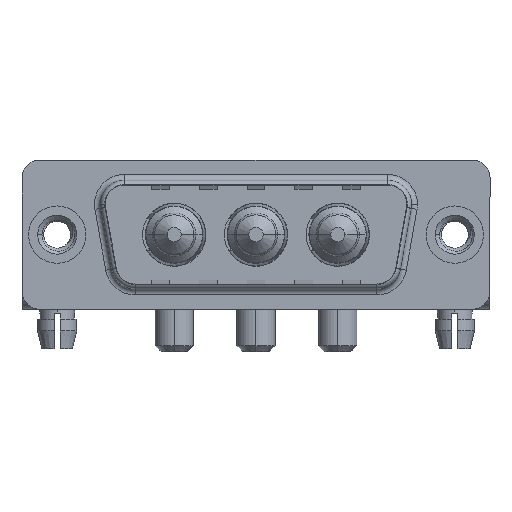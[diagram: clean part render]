
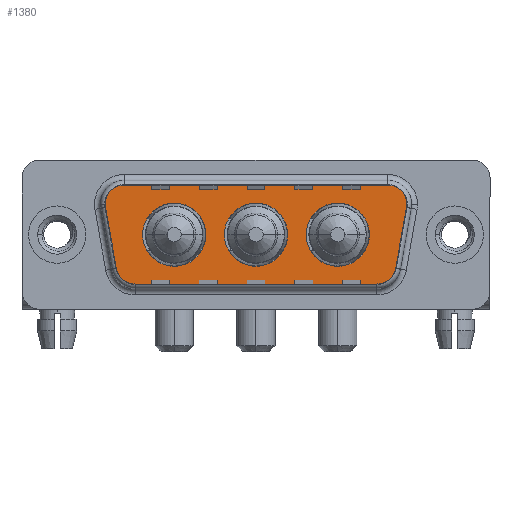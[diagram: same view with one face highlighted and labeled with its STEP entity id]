
A CAD part, top view. The second image highlights one B-rep face of the part: STEP entity #1380.
In plain terms, the highlighted planar face has unit normal (0, 0, 1).
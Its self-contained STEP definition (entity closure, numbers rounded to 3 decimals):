
#302 = DIRECTION ( 'NONE',  ( 0., 0., 1. ) ) ;
#380 = CARTESIAN_POINT ( 'NONE',  ( 26.866, -2.9, 0. ) ) ;
#477 = VECTOR ( 'NONE', #15163, 1000. ) ;
#493 = AXIS2_PLACEMENT_3D ( 'NONE', #7158, #10575, #11893 ) ;
#633 = VERTEX_POINT ( 'NONE', #14245 ) ;
#839 = EDGE_CURVE ( 'NONE', #13134, #1297, #13223, .T. ) ;
#893 = DIRECTION ( 'NONE',  ( -1., 0., 0. ) ) ;
#986 = DIRECTION ( 'NONE',  ( 1., 0., 0. ) ) ;
#1160 = VERTEX_POINT ( 'NONE', #13136 ) ;
#1214 = ORIENTED_EDGE ( 'NONE', *, *, #11689, .T. ) ;
#1252 = CIRCLE ( 'NONE', #4707, 2.65 ) ;
#1283 = DIRECTION ( 'NONE',  ( 0., 0., 1. ) ) ;
#1297 = VERTEX_POINT ( 'NONE', #1466 ) ;
#1345 = DIRECTION ( 'NONE',  ( 0., 0., 1. ) ) ;
#1366 = DIRECTION ( 'NONE',  ( 0., 0., 1. ) ) ;
#1380 = ADVANCED_FACE ( 'NONE', ( #2771, #7483, #3782, #6254 ), #10968, .T. ) ;
#1466 = CARTESIAN_POINT ( 'NONE',  ( 4.464, -3.247, 0. ) ) ;
#1900 = AXIS2_PLACEMENT_3D ( 'NONE', #6767, #10247, #986 ) ;
#2054 = ORIENTED_EDGE ( 'NONE', *, *, #5773, .F. ) ;
#2319 = VERTEX_POINT ( 'NONE', #10124 ) ;
#2365 = DIRECTION ( 'NONE',  ( 1., 0., 0. ) ) ;
#2606 = DIRECTION ( 'NONE',  ( 1., 0., 0. ) ) ;
#2658 = VECTOR ( 'NONE', #12943, 1000. ) ;
#2663 = DIRECTION ( 'NONE',  ( 0., 0., 1. ) ) ;
#2695 = ORIENTED_EDGE ( 'NONE', *, *, #8251, .F. ) ;
#2771 = FACE_BOUND ( 'NONE', #2846, .T. ) ;
#2846 = EDGE_LOOP ( 'NONE', ( #8643, #2695 ) ) ;
#3133 = CARTESIAN_POINT ( 'NONE',  ( 26.15, 0., 0. ) ) ;
#3180 = LINE ( 'NONE', #15089, #477 ) ;
#3241 = CARTESIAN_POINT ( 'NONE',  ( 14., 0., 0. ) ) ;
#3299 = EDGE_LOOP ( 'NONE', ( #7519, #13326, #3746, #1214, #10969, #6042, #6668, #4087, #4563 ) ) ;
#3429 = VERTEX_POINT ( 'NONE', #3133 ) ;
#3434 = VERTEX_POINT ( 'NONE', #14890 ) ;
#3510 = CARTESIAN_POINT ( 'NONE',  ( 9.8, 0., 0. ) ) ;
#3746 = ORIENTED_EDGE ( 'NONE', *, *, #10269, .T. ) ;
#3782 = FACE_BOUND ( 'NONE', #5805, .T. ) ;
#3991 = VECTOR ( 'NONE', #12380, 1000. ) ;
#4087 = ORIENTED_EDGE ( 'NONE', *, *, #6778, .T. ) ;
#4117 = AXIS2_PLACEMENT_3D ( 'NONE', #10049, #4189, #8894 ) ;
#4134 = CIRCLE ( 'NONE', #4387, 2.65 ) ;
#4189 = DIRECTION ( 'NONE',  ( 0., 0., 1. ) ) ;
#4387 = AXIS2_PLACEMENT_3D ( 'NONE', #14500, #2663, #6298 ) ;
#4513 = CIRCLE ( 'NONE', #9452, 2.65 ) ;
#4563 = ORIENTED_EDGE ( 'NONE', *, *, #6713, .T. ) ;
#4707 = AXIS2_PLACEMENT_3D ( 'NONE', #11364, #11443, #15074 ) ;
#5083 = AXIS2_PLACEMENT_3D ( 'NONE', #7715, #8865, #9946 ) ;
#5104 = CIRCLE ( 'NONE', #10549, 2.65 ) ;
#5110 = EDGE_CURVE ( 'NONE', #11005, #15207, #3180, .T. ) ;
#5317 = CARTESIAN_POINT ( 'NONE',  ( 29.859, 2.553, 0. ) ) ;
#5606 = CIRCLE ( 'NONE', #12028, 2. ) ;
#5612 = ORIENTED_EDGE ( 'NONE', *, *, #12303, .F. ) ;
#5619 = AXIS2_PLACEMENT_3D ( 'NONE', #10804, #302, #10657 ) ;
#5686 = DIRECTION ( 'NONE',  ( 0., 0., 1. ) ) ;
#5773 = EDGE_CURVE ( 'NONE', #3429, #2319, #13820, .T. ) ;
#5805 = EDGE_LOOP ( 'NONE', ( #7192, #5612 ) ) ;
#6042 = ORIENTED_EDGE ( 'NONE', *, *, #7007, .T. ) ;
#6254 = FACE_OUTER_BOUND ( 'NONE', #3299, .T. ) ;
#6298 = DIRECTION ( 'NONE',  ( 1., 0., 0. ) ) ;
#6511 = EDGE_CURVE ( 'NONE', #14499, #7944, #1252, .T. ) ;
#6583 = CIRCLE ( 'NONE', #4117, 2. ) ;
#6668 = ORIENTED_EDGE ( 'NONE', *, *, #839, .T. ) ;
#6713 = EDGE_CURVE ( 'NONE', #1160, #13533, #13273, .T. ) ;
#6767 = CARTESIAN_POINT ( 'NONE',  ( 5.411, 2.9, 0. ) ) ;
#6778 = EDGE_CURVE ( 'NONE', #1297, #1160, #10783, .T. ) ;
#6898 = LINE ( 'NONE', #14104, #2658 ) ;
#7007 = EDGE_CURVE ( 'NONE', #12529, #13134, #15237, .T. ) ;
#7013 = CARTESIAN_POINT ( 'NONE',  ( 6.434, -4.9, 0. ) ) ;
#7117 = EDGE_LOOP ( 'NONE', ( #2054, #9067 ) ) ;
#7158 = CARTESIAN_POINT ( 'NONE',  ( 23.5, 0., 0. ) ) ;
#7192 = ORIENTED_EDGE ( 'NONE', *, *, #7694, .F. ) ;
#7483 = FACE_BOUND ( 'NONE', #7117, .T. ) ;
#7519 = ORIENTED_EDGE ( 'NONE', *, *, #8624, .T. ) ;
#7694 = EDGE_CURVE ( 'NONE', #633, #3434, #4513, .T. ) ;
#7715 = CARTESIAN_POINT ( 'NONE',  ( 16.65, 0., 0. ) ) ;
#7944 = VERTEX_POINT ( 'NONE', #3241 ) ;
#8218 = DIRECTION ( 'NONE',  ( 1., 0., 0. ) ) ;
#8251 = EDGE_CURVE ( 'NONE', #7944, #14499, #11761, .T. ) ;
#8624 = EDGE_CURVE ( 'NONE', #13533, #11005, #11993, .T. ) ;
#8643 = ORIENTED_EDGE ( 'NONE', *, *, #6511, .F. ) ;
#8735 = CARTESIAN_POINT ( 'NONE',  ( 3.441, 2.553, 0. ) ) ;
#8807 = VECTOR ( 'NONE', #2606, 1000. ) ;
#8865 = DIRECTION ( 'NONE',  ( 0., 0., 1. ) ) ;
#8894 = DIRECTION ( 'NONE',  ( -1., 0., 0. ) ) ;
#9067 = ORIENTED_EDGE ( 'NONE', *, *, #12473, .F. ) ;
#9387 = DIRECTION ( 'NONE',  ( 1., 0., 0. ) ) ;
#9392 = VERTEX_POINT ( 'NONE', #14866 ) ;
#9397 = CARTESIAN_POINT ( 'NONE',  ( 9.8, 0., 0. ) ) ;
#9452 = AXIS2_PLACEMENT_3D ( 'NONE', #3510, #1345, #8218 ) ;
#9549 = CARTESIAN_POINT ( 'NONE',  ( 26.866, -2.9, 0. ) ) ;
#9691 = CARTESIAN_POINT ( 'NONE',  ( 3.441, 2.553, 0. ) ) ;
#9946 = DIRECTION ( 'NONE',  ( 1., 0., 0. ) ) ;
#9989 = CARTESIAN_POINT ( 'NONE',  ( 28.836, -3.247, 0. ) ) ;
#10049 = CARTESIAN_POINT ( 'NONE',  ( 27.889, 2.9, 0. ) ) ;
#10124 = CARTESIAN_POINT ( 'NONE',  ( 20.85, 0., 0. ) ) ;
#10152 = CARTESIAN_POINT ( 'NONE',  ( 5.411, 4.9, 0. ) ) ;
#10247 = DIRECTION ( 'NONE',  ( 0., 0., 1. ) ) ;
#10269 = EDGE_CURVE ( 'NONE', #15207, #9392, #5606, .T. ) ;
#10339 = VERTEX_POINT ( 'NONE', #10542 ) ;
#10542 = CARTESIAN_POINT ( 'NONE',  ( 27.889, 4.9, 0. ) ) ;
#10549 = AXIS2_PLACEMENT_3D ( 'NONE', #9397, #1283, #2365 ) ;
#10575 = DIRECTION ( 'NONE',  ( 0., 0., 1. ) ) ;
#10657 = DIRECTION ( 'NONE',  ( -1., 0., 0. ) ) ;
#10783 = CIRCLE ( 'NONE', #5619, 2. ) ;
#10804 = CARTESIAN_POINT ( 'NONE',  ( 6.434, -2.9, 0. ) ) ;
#10968 = PLANE ( 'NONE',  #13151 ) ;
#10969 = ORIENTED_EDGE ( 'NONE', *, *, #12852, .T. ) ;
#11005 = VERTEX_POINT ( 'NONE', #9989 ) ;
#11204 = CARTESIAN_POINT ( 'NONE',  ( 26.866, -4.9, 0. ) ) ;
#11364 = CARTESIAN_POINT ( 'NONE',  ( 16.65, 0., 0. ) ) ;
#11443 = DIRECTION ( 'NONE',  ( 0., 0., 1. ) ) ;
#11556 = CARTESIAN_POINT ( 'NONE',  ( 27.889, 2.9, 0. ) ) ;
#11689 = EDGE_CURVE ( 'NONE', #9392, #10339, #6583, .T. ) ;
#11761 = CIRCLE ( 'NONE', #5083, 2.65 ) ;
#11763 = CARTESIAN_POINT ( 'NONE',  ( 19.3, 0., 0. ) ) ;
#11893 = DIRECTION ( 'NONE',  ( 1., 0., 0. ) ) ;
#11993 = CIRCLE ( 'NONE', #14584, 2. ) ;
#12028 = AXIS2_PLACEMENT_3D ( 'NONE', #11556, #5686, #893 ) ;
#12209 = DIRECTION ( 'NONE',  ( 0., 0., 1. ) ) ;
#12303 = EDGE_CURVE ( 'NONE', #3434, #633, #5104, .T. ) ;
#12380 = DIRECTION ( 'NONE',  ( 0.174, -0.985, 0. ) ) ;
#12473 = EDGE_CURVE ( 'NONE', #2319, #3429, #4134, .T. ) ;
#12529 = VERTEX_POINT ( 'NONE', #10152 ) ;
#12852 = EDGE_CURVE ( 'NONE', #10339, #12529, #6898, .T. ) ;
#12943 = DIRECTION ( 'NONE',  ( -1., 0., 0. ) ) ;
#13134 = VERTEX_POINT ( 'NONE', #9691 ) ;
#13136 = CARTESIAN_POINT ( 'NONE',  ( 6.434, -4.9, 0. ) ) ;
#13151 = AXIS2_PLACEMENT_3D ( 'NONE', #380, #12209, #9387 ) ;
#13223 = LINE ( 'NONE', #8735, #3991 ) ;
#13273 = LINE ( 'NONE', #7013, #8807 ) ;
#13326 = ORIENTED_EDGE ( 'NONE', *, *, #5110, .T. ) ;
#13533 = VERTEX_POINT ( 'NONE', #11204 ) ;
#13820 = CIRCLE ( 'NONE', #493, 2.65 ) ;
#14104 = CARTESIAN_POINT ( 'NONE',  ( 5.411, 4.9, 0. ) ) ;
#14132 = DIRECTION ( 'NONE',  ( 1., 0., 0. ) ) ;
#14245 = CARTESIAN_POINT ( 'NONE',  ( 12.45, 0., 0. ) ) ;
#14499 = VERTEX_POINT ( 'NONE', #11763 ) ;
#14500 = CARTESIAN_POINT ( 'NONE',  ( 23.5, 0., 0. ) ) ;
#14584 = AXIS2_PLACEMENT_3D ( 'NONE', #9549, #1366, #14132 ) ;
#14866 = CARTESIAN_POINT ( 'NONE',  ( 29.889, 2.9, 0. ) ) ;
#14890 = CARTESIAN_POINT ( 'NONE',  ( 7.15, 0., 0. ) ) ;
#15074 = DIRECTION ( 'NONE',  ( 1., 0., 0. ) ) ;
#15089 = CARTESIAN_POINT ( 'NONE',  ( 29.859, 2.553, 0. ) ) ;
#15163 = DIRECTION ( 'NONE',  ( 0.174, 0.985, 0. ) ) ;
#15207 = VERTEX_POINT ( 'NONE', #5317 ) ;
#15237 = CIRCLE ( 'NONE', #1900, 2. ) ;
